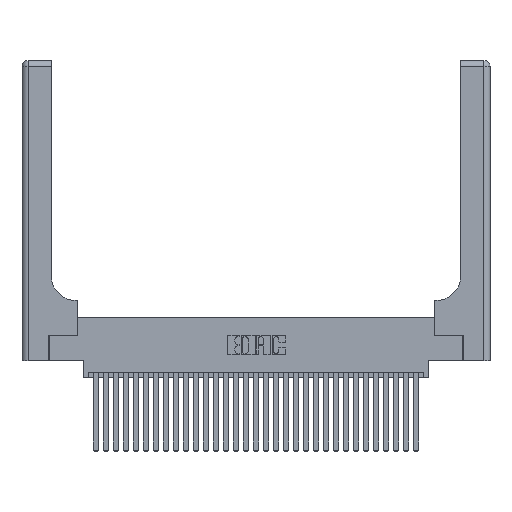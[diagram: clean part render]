
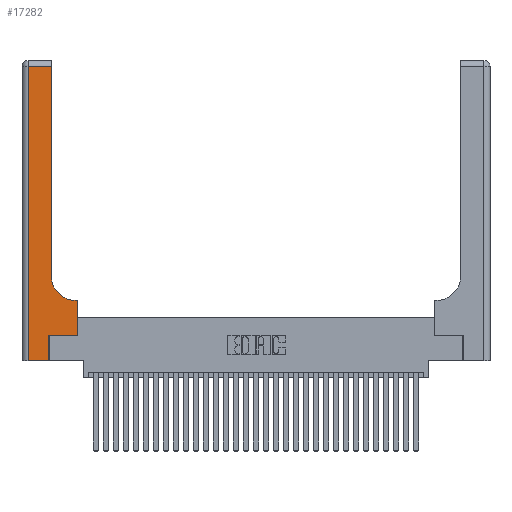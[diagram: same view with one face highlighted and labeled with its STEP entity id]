
A CAD part, top view. The second image highlights one B-rep face of the part: STEP entity #17282.
In plain terms, the highlighted planar face has unit normal (0, 0, 1).
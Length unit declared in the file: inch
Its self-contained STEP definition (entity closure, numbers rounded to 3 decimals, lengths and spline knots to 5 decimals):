
#1080 = ORIENTED_EDGE ( 'NONE', *, *, #4618, .T. ) ;
#1457 = PLANE ( 'NONE',  #29511 ) ;
#2498 = CARTESIAN_POINT ( 'NONE',  ( 0.06, 3., 0.37 ) ) ;
#2629 = CARTESIAN_POINT ( 'NONE',  ( 0., 0., 0.37 ) ) ;
#2644 = VERTEX_POINT ( 'NONE', #12458 ) ;
#3079 = CARTESIAN_POINT ( 'NONE',  ( 0.269, 0.25, 0.37 ) ) ;
#4312 = EDGE_CURVE ( 'NONE', #2644, #12192, #20848, .T. ) ;
#4618 = EDGE_CURVE ( 'NONE', #30718, #15812, #28197, .T. ) ;
#5767 = LINE ( 'NONE', #19905, #26839 ) ;
#6440 = LINE ( 'NONE', #32059, #19650 ) ;
#6763 = VERTEX_POINT ( 'NONE', #14682 ) ;
#7386 = VERTEX_POINT ( 'NONE', #32099 ) ;
#7559 = VECTOR ( 'NONE', #25524, 39.37008 ) ;
#7878 = CARTESIAN_POINT ( 'NONE',  ( 0.5585, 0.25, 0.37 ) ) ;
#8054 = EDGE_CURVE ( 'NONE', #15812, #7386, #28418, .T. ) ;
#8232 = VERTEX_POINT ( 'NONE', #18087 ) ;
#8621 = VERTEX_POINT ( 'NONE', #11255 ) ;
#9701 = LINE ( 'NONE', #7878, #13207 ) ;
#9878 = DIRECTION ( 'NONE',  ( 1., 0., 0. ) ) ;
#10183 = ORIENTED_EDGE ( 'NONE', *, *, #18289, .T. ) ;
#10458 = CARTESIAN_POINT ( 'NONE',  ( 0., 2.94, 0.37 ) ) ;
#10589 = CARTESIAN_POINT ( 'NONE',  ( 0.2915, 3., 0.37 ) ) ;
#10702 = LINE ( 'NONE', #17724, #11062 ) ;
#11062 = VECTOR ( 'NONE', #17939, 39.37008 ) ;
#11153 = CARTESIAN_POINT ( 'NONE',  ( 0.2915, 2.94, 0.37 ) ) ;
#11255 = CARTESIAN_POINT ( 'NONE',  ( 0.5585, 0.6, 0.37 ) ) ;
#11259 = CARTESIAN_POINT ( 'NONE',  ( 0.06, 2.94, 0.37 ) ) ;
#11356 = LINE ( 'NONE', #10458, #21497 ) ;
#11427 = DIRECTION ( 'NONE',  ( -1., 0., 0. ) ) ;
#11488 = EDGE_CURVE ( 'NONE', #12192, #30718, #11356, .T. ) ;
#12192 = VERTEX_POINT ( 'NONE', #11153 ) ;
#12458 = CARTESIAN_POINT ( 'NONE',  ( 0.2915, 0.85, 0.37 ) ) ;
#13207 = VECTOR ( 'NONE', #15654, 39.37008 ) ;
#14682 = CARTESIAN_POINT ( 'NONE',  ( 0.5585, 0.25, 0.37 ) ) ;
#14775 = CIRCLE ( 'NONE', #30388, 0.25 ) ;
#15654 = DIRECTION ( 'NONE',  ( 0., 1., 0. ) ) ;
#15712 = DIRECTION ( 'NONE',  ( -1., 0., 0. ) ) ;
#15800 = CARTESIAN_POINT ( 'NONE',  ( 0.5415, 0.85, 0.37 ) ) ;
#15812 = VERTEX_POINT ( 'NONE', #23334 ) ;
#16556 = ORIENTED_EDGE ( 'NONE', *, *, #24888, .T. ) ;
#16788 = ORIENTED_EDGE ( 'NONE', *, *, #4312, .T. ) ;
#17282 = ADVANCED_FACE ( 'NONE', ( #28837 ), #1457, .F. ) ;
#17724 = CARTESIAN_POINT ( 'NONE',  ( 0.269, 0., 0.37 ) ) ;
#17819 = EDGE_CURVE ( 'NONE', #8232, #2644, #14775, .T. ) ;
#17939 = DIRECTION ( 'NONE',  ( 0., 1., 0. ) ) ;
#18087 = CARTESIAN_POINT ( 'NONE',  ( 0.5415, 0.6, 0.37 ) ) ;
#18289 = EDGE_CURVE ( 'NONE', #22621, #6763, #5767, .T. ) ;
#18608 = EDGE_LOOP ( 'NONE', ( #16788, #26434, #1080, #26626, #28720, #10183, #16556, #30133, #23427 ) ) ;
#19650 = VECTOR ( 'NONE', #27165, 39.37008 ) ;
#19905 = CARTESIAN_POINT ( 'NONE',  ( 0.269, 0.25, 0.37 ) ) ;
#20799 = DIRECTION ( 'NONE',  ( 1., 0., 0. ) ) ;
#20848 = LINE ( 'NONE', #10589, #7559 ) ;
#21497 = VECTOR ( 'NONE', #15712, 39.37008 ) ;
#21796 = VECTOR ( 'NONE', #9878, 39.37008 ) ;
#22621 = VERTEX_POINT ( 'NONE', #3079 ) ;
#22773 = VECTOR ( 'NONE', #29899, 39.37008 ) ;
#23334 = CARTESIAN_POINT ( 'NONE',  ( 0.06, 0., 0.37 ) ) ;
#23427 = ORIENTED_EDGE ( 'NONE', *, *, #17819, .T. ) ;
#24888 = EDGE_CURVE ( 'NONE', #6763, #8621, #9701, .T. ) ;
#25524 = DIRECTION ( 'NONE',  ( 0., 1., 0. ) ) ;
#26434 = ORIENTED_EDGE ( 'NONE', *, *, #11488, .T. ) ;
#26626 = ORIENTED_EDGE ( 'NONE', *, *, #8054, .T. ) ;
#26839 = VECTOR ( 'NONE', #27626, 39.37008 ) ;
#27165 = DIRECTION ( 'NONE',  ( -1., 0., 0. ) ) ;
#27626 = DIRECTION ( 'NONE',  ( 1., 0., 0. ) ) ;
#28197 = LINE ( 'NONE', #2498, #22773 ) ;
#28353 = EDGE_CURVE ( 'NONE', #7386, #22621, #10702, .T. ) ;
#28418 = LINE ( 'NONE', #2629, #21796 ) ;
#28720 = ORIENTED_EDGE ( 'NONE', *, *, #28353, .T. ) ;
#28837 = FACE_OUTER_BOUND ( 'NONE', #18608, .T. ) ;
#29138 = EDGE_CURVE ( 'NONE', #8621, #8232, #6440, .T. ) ;
#29511 = AXIS2_PLACEMENT_3D ( 'NONE', #31357, #31250, #11427 ) ;
#29899 = DIRECTION ( 'NONE',  ( 0., -1., 0. ) ) ;
#30133 = ORIENTED_EDGE ( 'NONE', *, *, #29138, .T. ) ;
#30379 = DIRECTION ( 'NONE',  ( 0., 0., -1. ) ) ;
#30388 = AXIS2_PLACEMENT_3D ( 'NONE', #15800, #30379, #20799 ) ;
#30718 = VERTEX_POINT ( 'NONE', #11259 ) ;
#31250 = DIRECTION ( 'NONE',  ( 0., 0., -1. ) ) ;
#31357 = CARTESIAN_POINT ( 'NONE',  ( 0., 3., 0.37 ) ) ;
#32059 = CARTESIAN_POINT ( 'NONE',  ( 0.2915, 0.6, 0.37 ) ) ;
#32099 = CARTESIAN_POINT ( 'NONE',  ( 0.269, 0., 0.37 ) ) ;
